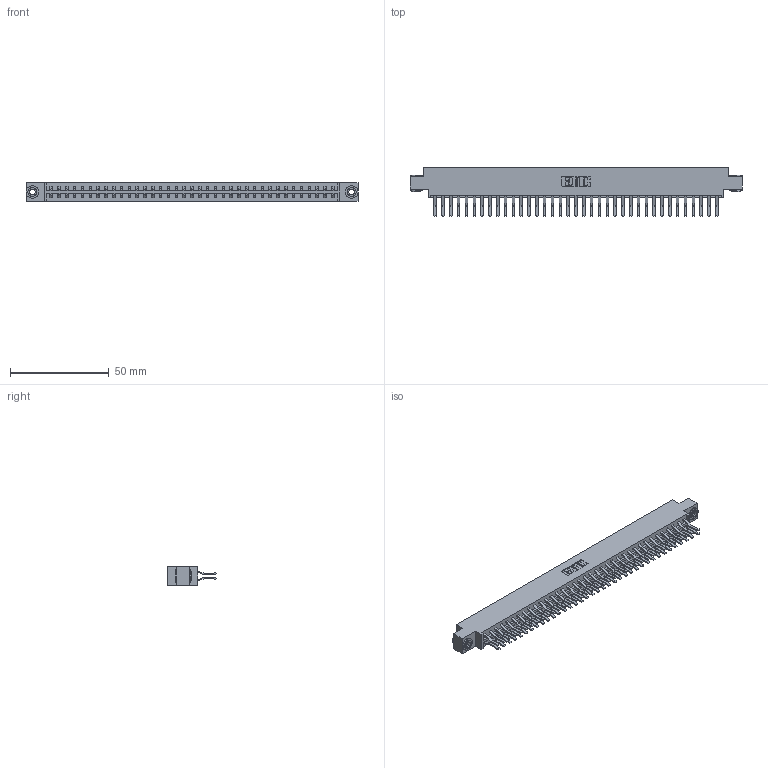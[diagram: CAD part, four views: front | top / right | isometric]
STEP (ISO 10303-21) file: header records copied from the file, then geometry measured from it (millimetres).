
FILE_DESCRIPTION (( 'STEP AP203' ), '1' );
FILE_NAME ('333-074-560-803.STEP', '2018-08-04T22:30:32', ( '' ), ( '' ), 'SwSTEP 2.0', 'SolidWorks 2016', '' );
FILE_SCHEMA (( 'CONFIG_CONTROL_DESIGN' ));
Length unit declared in the file: inch
Products named in the file (4): 333 Part_Offset - .156 Dia - TH; 345-292-001_560 Tail; 345-250-002_345-250-002-102; 333-074-560-803
Assembly tree (77 placements, depth 2):
  333-074-560-803
    333 Part_Offset - .156 Dia - TH
    345-292-001_560 Tail  x74
    345-250-002_345-250-002-102  x2
Bounding box: 168.15 x 24.78 x 9.4 mm (x, y, z)
Volume: 17396.8 mm3; surface area: 22339 mm2
Topology: 77 solids, 77 shells, 4152 faces, 12313 edges, 8106 vertices
Faces by surface type: plane 2748, cylinder 1396, cone 8
Entity records: 25320 total; most frequent: CARTESIAN_POINT 4181, ORIENTED_EDGE 4110, DIRECTION 3617, EDGE_CURVE 2055, LINE 1899, VECTOR 1899, VERTEX_POINT 1366, AXIS2_PLACEMENT_3D 859
